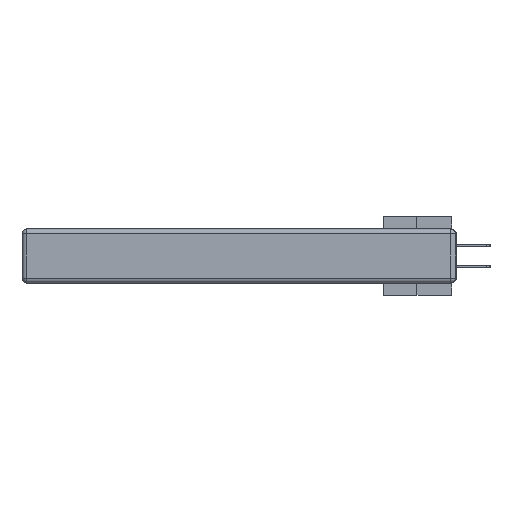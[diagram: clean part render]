
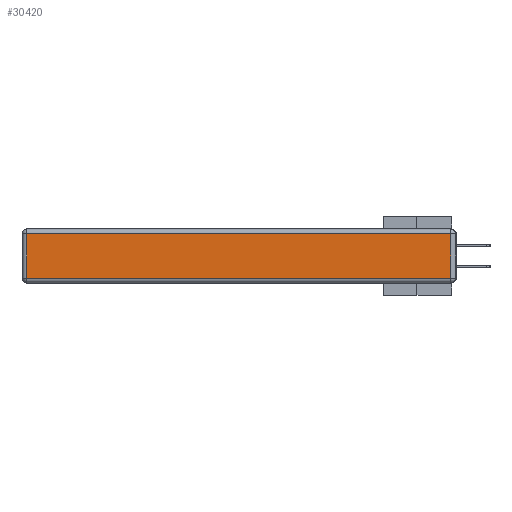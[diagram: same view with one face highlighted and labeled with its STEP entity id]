
A CAD part, left-side view. The second image highlights one B-rep face of the part: STEP entity #30420.
In plain terms, the highlighted planar face has unit normal (-1, 0, 0).
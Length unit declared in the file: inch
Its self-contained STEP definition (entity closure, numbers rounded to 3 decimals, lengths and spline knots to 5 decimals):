
#2454 = DIRECTION ( 'NONE',  ( 0., 0., 1. ) ) ;
#2831 = VECTOR ( 'NONE', #9221, 39.37008 ) ;
#3008 = DIRECTION ( 'NONE',  ( -1., 0., 0. ) ) ;
#3044 = CARTESIAN_POINT ( 'NONE',  ( 0., 2.72, -0.313 ) ) ;
#3148 = DIRECTION ( 'NONE',  ( 0., 0., -1. ) ) ;
#3338 = VECTOR ( 'NONE', #27885, 39.37008 ) ;
#4247 = ORIENTED_EDGE ( 'NONE', *, *, #18591, .T. ) ;
#5304 = CARTESIAN_POINT ( 'NONE',  ( 0., 2.72, -0.03 ) ) ;
#5458 = CARTESIAN_POINT ( 'NONE',  ( 0., 0.03, -0.313 ) ) ;
#8106 = ORIENTED_EDGE ( 'NONE', *, *, #24805, .T. ) ;
#9221 = DIRECTION ( 'NONE',  ( 0., 1., 0. ) ) ;
#10299 = LINE ( 'NONE', #32783, #28408 ) ;
#10879 = EDGE_LOOP ( 'NONE', ( #4247, #8106, #35768, #13144 ) ) ;
#13144 = ORIENTED_EDGE ( 'NONE', *, *, #32189, .T. ) ;
#17194 = LINE ( 'NONE', #27021, #2831 ) ;
#17602 = CARTESIAN_POINT ( 'NONE',  ( 0., 0.03, -0.343 ) ) ;
#18168 = LINE ( 'NONE', #18477, #3338 ) ;
#18477 = CARTESIAN_POINT ( 'NONE',  ( 0., 0., -0.313 ) ) ;
#18591 = EDGE_CURVE ( 'NONE', #29348, #26305, #18168, .T. ) ;
#21486 = VERTEX_POINT ( 'NONE', #5304 ) ;
#22512 = CARTESIAN_POINT ( 'NONE',  ( 0., 0.03, -0.03 ) ) ;
#23776 = DIRECTION ( 'NONE',  ( 0., 0., 1. ) ) ;
#24805 = EDGE_CURVE ( 'NONE', #26305, #29831, #33202, .T. ) ;
#26305 = VERTEX_POINT ( 'NONE', #5458 ) ;
#27021 = CARTESIAN_POINT ( 'NONE',  ( 0., 2.75, -0.03 ) ) ;
#27885 = DIRECTION ( 'NONE',  ( 0., -1., 0. ) ) ;
#28408 = VECTOR ( 'NONE', #3148, 39.37008 ) ;
#29348 = VERTEX_POINT ( 'NONE', #3044 ) ;
#29831 = VERTEX_POINT ( 'NONE', #22512 ) ;
#30401 = AXIS2_PLACEMENT_3D ( 'NONE', #35495, #3008, #23776 ) ;
#30403 = VECTOR ( 'NONE', #2454, 39.37008 ) ;
#30420 = ADVANCED_FACE ( 'NONE', ( #33627 ), #38332, .T. ) ;
#32189 = EDGE_CURVE ( 'NONE', #21486, #29348, #10299, .T. ) ;
#32783 = CARTESIAN_POINT ( 'NONE',  ( 0., 2.72, -0.343 ) ) ;
#33202 = LINE ( 'NONE', #17602, #30403 ) ;
#33627 = FACE_OUTER_BOUND ( 'NONE', #10879, .T. ) ;
#35495 = CARTESIAN_POINT ( 'NONE',  ( 0., 0., -0.343 ) ) ;
#35768 = ORIENTED_EDGE ( 'NONE', *, *, #37809, .T. ) ;
#37809 = EDGE_CURVE ( 'NONE', #29831, #21486, #17194, .T. ) ;
#38332 = PLANE ( 'NONE',  #30401 ) ;
